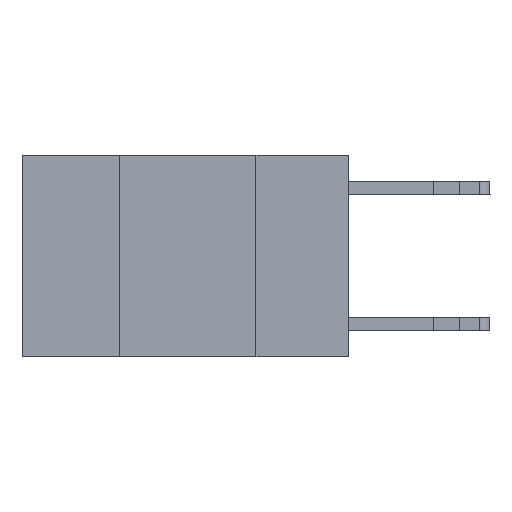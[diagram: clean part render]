
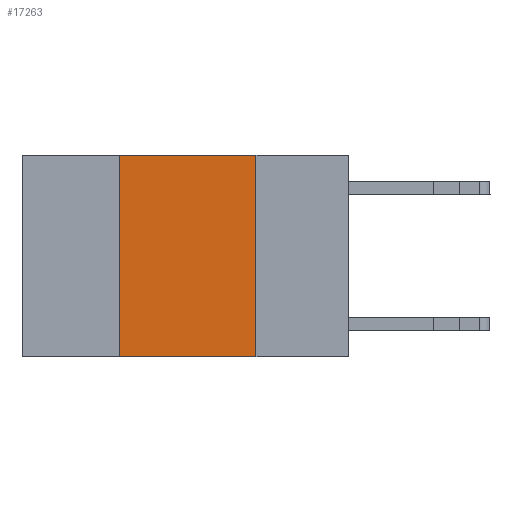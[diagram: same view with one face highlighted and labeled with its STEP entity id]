
A CAD part, left-side view. The second image highlights one B-rep face of the part: STEP entity #17263.
In plain terms, the highlighted planar face has unit normal (-1, 0, 0).
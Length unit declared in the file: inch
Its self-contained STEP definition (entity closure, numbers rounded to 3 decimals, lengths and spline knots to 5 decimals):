
#807 = EDGE_CURVE ( 'NONE', #23661, #5121, #1617, .T. ) ;
#1404 = VECTOR ( 'NONE', #7404, 39.37008 ) ;
#1617 = LINE ( 'NONE', #6548, #1404 ) ;
#2217 = AXIS2_PLACEMENT_3D ( 'NONE', #15449, #11611, #10849 ) ;
#2752 = VECTOR ( 'NONE', #23866, 39.37008 ) ;
#2869 = LINE ( 'NONE', #24021, #2752 ) ;
#4058 = EDGE_LOOP ( 'NONE', ( #16165, #8478, #8580, #8882 ) ) ;
#5121 = VERTEX_POINT ( 'NONE', #15724 ) ;
#5583 = CARTESIAN_POINT ( 'NONE',  ( 0., 0.42, 0. ) ) ;
#6548 = CARTESIAN_POINT ( 'NONE',  ( 0., 0.6, -0.37 ) ) ;
#6995 = VERTEX_POINT ( 'NONE', #5583 ) ;
#7182 = EDGE_CURVE ( 'NONE', #23997, #5121, #2869, .T. ) ;
#7404 = DIRECTION ( 'NONE',  ( 0., -1., 0. ) ) ;
#7732 = EDGE_CURVE ( 'NONE', #6995, #23997, #12670, .T. ) ;
#8478 = ORIENTED_EDGE ( 'NONE', *, *, #7732, .F. ) ;
#8580 = ORIENTED_EDGE ( 'NONE', *, *, #20152, .F. ) ;
#8815 = CARTESIAN_POINT ( 'NONE',  ( 0., 0.17, 0. ) ) ;
#8882 = ORIENTED_EDGE ( 'NONE', *, *, #807, .T. ) ;
#9645 = PLANE ( 'NONE',  #2217 ) ;
#10849 = DIRECTION ( 'NONE',  ( 0., 0., -1. ) ) ;
#11284 = DIRECTION ( 'NONE',  ( 0., 0., 1. ) ) ;
#11573 = FACE_OUTER_BOUND ( 'NONE', #4058, .T. ) ;
#11611 = DIRECTION ( 'NONE',  ( 1., 0., 0. ) ) ;
#12670 = LINE ( 'NONE', #16749, #12903 ) ;
#12903 = VECTOR ( 'NONE', #16671, 39.37008 ) ;
#15086 = VECTOR ( 'NONE', #11284, 39.37008 ) ;
#15165 = LINE ( 'NONE', #22426, #15086 ) ;
#15449 = CARTESIAN_POINT ( 'NONE',  ( 0., 0.6, 0. ) ) ;
#15724 = CARTESIAN_POINT ( 'NONE',  ( 0., 0.17, -0.37 ) ) ;
#16165 = ORIENTED_EDGE ( 'NONE', *, *, #7182, .F. ) ;
#16671 = DIRECTION ( 'NONE',  ( 0., -1., 0. ) ) ;
#16749 = CARTESIAN_POINT ( 'NONE',  ( 0., 0.6, 0. ) ) ;
#17263 = ADVANCED_FACE ( 'NONE', ( #11573 ), #9645, .F. ) ;
#20152 = EDGE_CURVE ( 'NONE', #23661, #6995, #15165, .T. ) ;
#22426 = CARTESIAN_POINT ( 'NONE',  ( 0., 0.42, 0. ) ) ;
#22921 = CARTESIAN_POINT ( 'NONE',  ( 0., 0.42, -0.37 ) ) ;
#23661 = VERTEX_POINT ( 'NONE', #22921 ) ;
#23866 = DIRECTION ( 'NONE',  ( 0., 0., -1. ) ) ;
#23997 = VERTEX_POINT ( 'NONE', #8815 ) ;
#24021 = CARTESIAN_POINT ( 'NONE',  ( 0., 0.17, 0. ) ) ;
